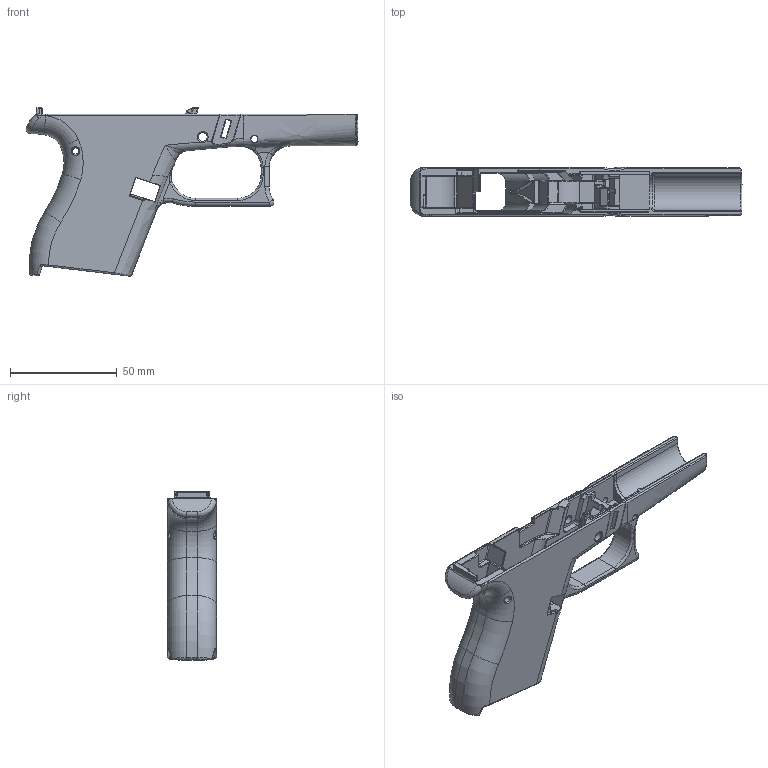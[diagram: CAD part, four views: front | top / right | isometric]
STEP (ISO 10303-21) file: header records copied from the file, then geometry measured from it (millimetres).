
FILE_DESCRIPTION(/* description */ (''),/* implementation_level */ '2;1');
FILE_NAME(/* name */ 'Frame OEM (ChairmanWon).step',/* time_stamp */ '2022-01-02T17:22:16-05:00',/* author */ (''),/* organization */ (''),/* preprocessor_version */ 'ST-DEVELOPER v18.1',/* originating_system */ 'Autodesk Translation Framework v10.10.0.1391',/* authorisation */ '');
FILE_SCHEMA (('AUTOMOTIVE_DESIGN { 1 0 10303 214 3 1 1 }'));
Products named in the file (1): Frame OEM (ChairmanWon)
Bounding box: 155.83 x 23 x 79.07 mm (x, y, z)
Volume: 47980.4 mm3; surface area: 31436.9 mm2
Topology: 1 solids, 1 shells, 929 faces, 2400 edges, 1420 vertices
Faces by surface type: cylinder 308, bspline 292, plane 183, torus 84, sphere 39, cone 23
Full cylindrical faces by diameter (mm): 3.05 x2, 3.3 x2, 3.5 x1, 4.25 x2
Entity records: 48207 total; most frequent: CARTESIAN_POINT 27528, ORIENTED_EDGE 4716, DIRECTION 3804, EDGE_CURVE 2358, AXIS2_PLACEMENT_3D 1478, VERTEX_POINT 1419, EDGE_LOOP 941, FACE_OUTER_BOUND 928
